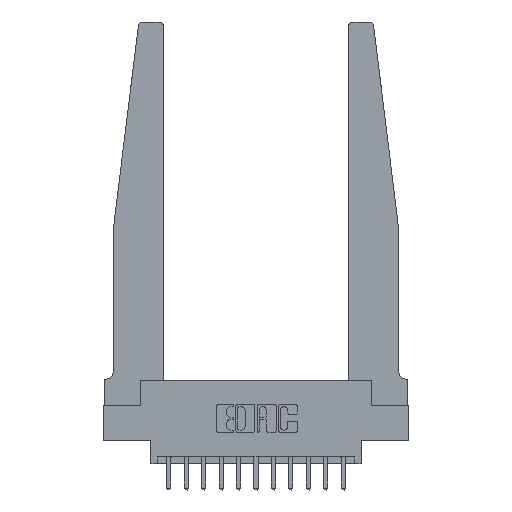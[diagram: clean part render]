
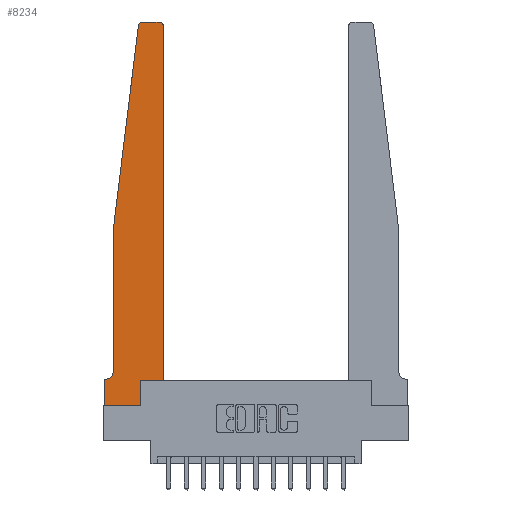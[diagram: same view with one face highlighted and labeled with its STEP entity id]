
A CAD part, top view. The second image highlights one B-rep face of the part: STEP entity #8234.
In plain terms, the highlighted planar face has unit normal (0, 0, 1).
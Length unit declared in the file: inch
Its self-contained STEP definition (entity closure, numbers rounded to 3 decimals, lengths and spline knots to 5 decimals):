
#275 = VECTOR ( 'NONE', #13900, 39.37008 ) ;
#352 = EDGE_CURVE ( 'NONE', #11758, #16032, #10825, .T. ) ;
#441 = CARTESIAN_POINT ( 'NONE',  ( 0.425, 0.18, 0.37 ) ) ;
#530 = VECTOR ( 'NONE', #12437, 39.37008 ) ;
#572 = ORIENTED_EDGE ( 'NONE', *, *, #10908, .T. ) ;
#810 = CARTESIAN_POINT ( 'NONE',  ( 0.27653, 2.75, 0.37 ) ) ;
#1669 = DIRECTION ( 'NONE',  ( -1., 0., 0. ) ) ;
#1856 = CARTESIAN_POINT ( 'NONE',  ( 0.2605, 0.18, 0.37 ) ) ;
#2056 = ORIENTED_EDGE ( 'NONE', *, *, #15931, .T. ) ;
#2082 = LINE ( 'NONE', #7284, #530 ) ;
#2288 = VECTOR ( 'NONE', #9296, 39.37008 ) ;
#2584 = DIRECTION ( 'NONE',  ( 0., 0., 1. ) ) ;
#2798 = EDGE_CURVE ( 'NONE', #12517, #4151, #2082, .T. ) ;
#3370 = ORIENTED_EDGE ( 'NONE', *, *, #2798, .T. ) ;
#3471 = VERTEX_POINT ( 'NONE', #16224 ) ;
#3594 = EDGE_CURVE ( 'NONE', #4733, #12702, #13581, .T. ) ;
#3683 = VECTOR ( 'NONE', #8976, 39.37008 ) ;
#3824 = AXIS2_PLACEMENT_3D ( 'NONE', #7493, #12385, #11120 ) ;
#3974 = CARTESIAN_POINT ( 'NONE',  ( 0.015, 0.1875, 0.37 ) ) ;
#4121 = CARTESIAN_POINT ( 'NONE',  ( 0.065, 1.25, 0.37 ) ) ;
#4127 = EDGE_CURVE ( 'NONE', #16032, #8535, #13738, .T. ) ;
#4151 = VERTEX_POINT ( 'NONE', #810 ) ;
#4299 = CARTESIAN_POINT ( 'NONE',  ( 0.065, 0.1875, 0.37 ) ) ;
#4380 = CARTESIAN_POINT ( 'NONE',  ( 0., 0., 0.37 ) ) ;
#4382 = AXIS2_PLACEMENT_3D ( 'NONE', #8962, #15218, #15301 ) ;
#4516 = EDGE_CURVE ( 'NONE', #3471, #4733, #10307, .T. ) ;
#4596 = EDGE_CURVE ( 'NONE', #8535, #12517, #7659, .T. ) ;
#4733 = VERTEX_POINT ( 'NONE', #5484 ) ;
#4893 = CARTESIAN_POINT ( 'NONE',  ( 0.425, 2.72, 0.37 ) ) ;
#4896 = CARTESIAN_POINT ( 'NONE',  ( 0.27653, 2.72, 0.37 ) ) ;
#5079 = CIRCLE ( 'NONE', #11567, 0.03 ) ;
#5460 = ORIENTED_EDGE ( 'NONE', *, *, #16118, .T. ) ;
#5484 = CARTESIAN_POINT ( 'NONE',  ( 0.065, 0.2375, 0.37 ) ) ;
#5540 = CARTESIAN_POINT ( 'NONE',  ( 0.395, 2.75, 0.37 ) ) ;
#6043 = VECTOR ( 'NONE', #15478, 39.37008 ) ;
#6181 = DIRECTION ( 'NONE',  ( 1., 0., 0. ) ) ;
#6195 = ORIENTED_EDGE ( 'NONE', *, *, #7672, .T. ) ;
#7284 = CARTESIAN_POINT ( 'NONE',  ( 0.25, 2.75, 0.37 ) ) ;
#7493 = CARTESIAN_POINT ( 'NONE',  ( 0.015, 0.2375, 0.37 ) ) ;
#7623 = CARTESIAN_POINT ( 'NONE',  ( 0., 0., 0.37 ) ) ;
#7659 = CIRCLE ( 'NONE', #4382, 0.03 ) ;
#7672 = EDGE_CURVE ( 'NONE', #11948, #3471, #15743, .T. ) ;
#7697 = LINE ( 'NONE', #12859, #14472 ) ;
#7720 = CARTESIAN_POINT ( 'NONE',  ( 0., 0.1875, 0.37 ) ) ;
#8131 = CARTESIAN_POINT ( 'NONE',  ( 0.425, 0.18, 0.37 ) ) ;
#8149 = VECTOR ( 'NONE', #1669, 39.37008 ) ;
#8234 = ADVANCED_FACE ( 'NONE', ( #16785 ), #15414, .T. ) ;
#8362 = CARTESIAN_POINT ( 'NONE',  ( 0.2605, 0., 0.37 ) ) ;
#8535 = VERTEX_POINT ( 'NONE', #4893 ) ;
#8679 = EDGE_CURVE ( 'NONE', #16449, #11758, #7697, .T. ) ;
#8769 = ORIENTED_EDGE ( 'NONE', *, *, #4127, .T. ) ;
#8962 = CARTESIAN_POINT ( 'NONE',  ( 0.395, 2.72, 0.37 ) ) ;
#8976 = DIRECTION ( 'NONE',  ( 1., 0., 0. ) ) ;
#9045 = DIRECTION ( 'NONE',  ( 0., 1., 0. ) ) ;
#9296 = DIRECTION ( 'NONE',  ( -0.122, -0.992, 0. ) ) ;
#9554 = DIRECTION ( 'NONE',  ( 0., -1., 0. ) ) ;
#9839 = VERTEX_POINT ( 'NONE', #13030 ) ;
#9971 = CARTESIAN_POINT ( 'NONE',  ( 0.24675, 2.72367, 0.37 ) ) ;
#10001 = CARTESIAN_POINT ( 'NONE',  ( 0., 0., 0.37 ) ) ;
#10113 = AXIS2_PLACEMENT_3D ( 'NONE', #7720, #16608, #10160 ) ;
#10160 = DIRECTION ( 'NONE',  ( 1., 0., 0. ) ) ;
#10301 = ORIENTED_EDGE ( 'NONE', *, *, #4516, .T. ) ;
#10307 = LINE ( 'NONE', #16757, #6043 ) ;
#10825 = LINE ( 'NONE', #8131, #13243 ) ;
#10908 = EDGE_CURVE ( 'NONE', #15671, #16449, #14039, .T. ) ;
#11120 = DIRECTION ( 'NONE',  ( -1., 0., 0. ) ) ;
#11567 = AXIS2_PLACEMENT_3D ( 'NONE', #4896, #2584, #6181 ) ;
#11758 = VERTEX_POINT ( 'NONE', #1856 ) ;
#11775 = ORIENTED_EDGE ( 'NONE', *, *, #12085, .T. ) ;
#11895 = ORIENTED_EDGE ( 'NONE', *, *, #8679, .T. ) ;
#11948 = VERTEX_POINT ( 'NONE', #9971 ) ;
#12085 = EDGE_CURVE ( 'NONE', #4151, #11948, #5079, .T. ) ;
#12385 = DIRECTION ( 'NONE',  ( 0., 0., -1. ) ) ;
#12437 = DIRECTION ( 'NONE',  ( -1., 0., 0. ) ) ;
#12517 = VERTEX_POINT ( 'NONE', #5540 ) ;
#12702 = VERTEX_POINT ( 'NONE', #3974 ) ;
#12790 = ORIENTED_EDGE ( 'NONE', *, *, #3594, .T. ) ;
#12845 = EDGE_LOOP ( 'NONE', ( #3370, #11775, #6195, #10301, #12790, #2056, #5460, #572, #11895, #15846, #8769, #13656 ) ) ;
#12859 = CARTESIAN_POINT ( 'NONE',  ( 0.2605, 0.18, 0.37 ) ) ;
#13030 = CARTESIAN_POINT ( 'NONE',  ( 0., 0.1875, 0.37 ) ) ;
#13043 = CARTESIAN_POINT ( 'NONE',  ( 0.425, 0.18, 0.37 ) ) ;
#13243 = VECTOR ( 'NONE', #15838, 39.37008 ) ;
#13291 = LINE ( 'NONE', #4299, #8149 ) ;
#13581 = CIRCLE ( 'NONE', #3824, 0.05 ) ;
#13656 = ORIENTED_EDGE ( 'NONE', *, *, #4596, .T. ) ;
#13738 = LINE ( 'NONE', #13043, #275 ) ;
#13900 = DIRECTION ( 'NONE',  ( 0., 1., 0. ) ) ;
#14039 = LINE ( 'NONE', #7623, #3683 ) ;
#14472 = VECTOR ( 'NONE', #9045, 39.37008 ) ;
#15218 = DIRECTION ( 'NONE',  ( 0., 0., 1. ) ) ;
#15301 = DIRECTION ( 'NONE',  ( 1., 0., 0. ) ) ;
#15414 = PLANE ( 'NONE',  #10113 ) ;
#15478 = DIRECTION ( 'NONE',  ( 0., -1., 0. ) ) ;
#15671 = VERTEX_POINT ( 'NONE', #10001 ) ;
#15743 = LINE ( 'NONE', #4121, #2288 ) ;
#15838 = DIRECTION ( 'NONE',  ( 1., 0., 0. ) ) ;
#15846 = ORIENTED_EDGE ( 'NONE', *, *, #352, .T. ) ;
#15931 = EDGE_CURVE ( 'NONE', #12702, #9839, #13291, .T. ) ;
#15990 = VECTOR ( 'NONE', #9554, 39.37008 ) ;
#15996 = LINE ( 'NONE', #4380, #15990 ) ;
#16032 = VERTEX_POINT ( 'NONE', #441 ) ;
#16118 = EDGE_CURVE ( 'NONE', #9839, #15671, #15996, .T. ) ;
#16224 = CARTESIAN_POINT ( 'NONE',  ( 0.065, 1.25, 0.37 ) ) ;
#16449 = VERTEX_POINT ( 'NONE', #8362 ) ;
#16608 = DIRECTION ( 'NONE',  ( 0., 0., 1. ) ) ;
#16757 = CARTESIAN_POINT ( 'NONE',  ( 0.065, 1.25, 0.37 ) ) ;
#16785 = FACE_OUTER_BOUND ( 'NONE', #12845, .T. ) ;
